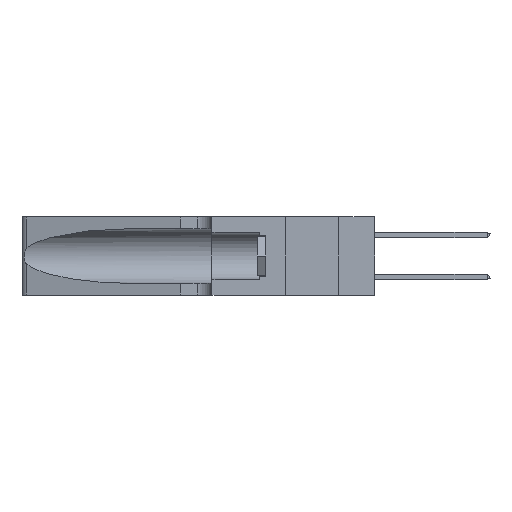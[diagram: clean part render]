
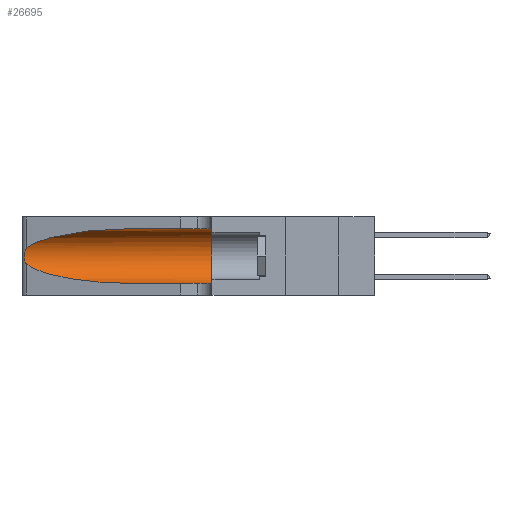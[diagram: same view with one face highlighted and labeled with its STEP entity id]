
A CAD part, left-side view. The second image highlights one B-rep face of the part: STEP entity #26695.
In plain terms, the highlighted cylindrical face has radius 3.308 mm (diameter 6.617 mm), a partial arc.
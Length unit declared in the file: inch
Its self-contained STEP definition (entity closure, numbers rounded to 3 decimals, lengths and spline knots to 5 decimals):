
#45 = VECTOR ( 'NONE', #2268, 39.37008 ) ;
#107 = VERTEX_POINT ( 'NONE', #2009 ) ;
#202 = DIRECTION ( 'NONE',  ( 0., -1., 0. ) ) ;
#942 = CARTESIAN_POINT ( 'NONE',  ( 0.25487, 1.22718, 0.14631 ) ) ;
#1218 = DIRECTION ( 'NONE',  ( 0., 0., 1. ) ) ;
#1444 = CARTESIAN_POINT ( 'NONE',  ( 0.25639, 1.23186, 0.15144 ) ) ;
#2009 = CARTESIAN_POINT ( 'NONE',  ( 0.1305, 0.72297, 0.05475 ) ) ;
#2268 = DIRECTION ( 'NONE',  ( 0., -1., 0. ) ) ;
#2345 = EDGE_CURVE ( 'NONE', #10786, #5442, #5849, .T. ) ;
#3218 = DIRECTION ( 'NONE',  ( 0., 1., 0. ) ) ;
#4179 = EDGE_CURVE ( 'NONE', #23238, #16284, #18968, .T. ) ;
#4226 = ORIENTED_EDGE ( 'NONE', *, *, #7872, .T. ) ;
#5297 = CARTESIAN_POINT ( 'NONE',  ( 0.25787, 1.23484, 0.2124 ) ) ;
#5377 =( BOUNDED_CURVE ( )  B_SPLINE_CURVE ( 3, ( #12181, #7871, #12654, #19190 ),
 .UNSPECIFIED., .F., .T. ) 
 B_SPLINE_CURVE_WITH_KNOTS ( ( 4, 4 ),
 ( 3.44316, 4.71239 ),
 .UNSPECIFIED. ) 
 CURVE ( )  GEOMETRIC_REPRESENTATION_ITEM ( )  RATIONAL_B_SPLINE_CURVE ( ( 1., 0.87, 0.87, 1. ) ) 
 REPRESENTATION_ITEM ( '' )  );
#5442 = VERTEX_POINT ( 'NONE', #18448 ) ;
#5849 = LINE ( 'NONE', #19438, #45 ) ;
#6917 = CARTESIAN_POINT ( 'NONE',  ( 0.25639, 1.23184, 0.21858 ) ) ;
#7208 = CIRCLE ( 'NONE', #15430, 0.13025 ) ;
#7463 = CYLINDRICAL_SURFACE ( 'NONE', #18417, 0.13025 ) ;
#7635 = CARTESIAN_POINT ( 'NONE',  ( 0.26075, 1.23896, 0.19203 ) ) ;
#7871 = CARTESIAN_POINT ( 'NONE',  ( 0.2373, 1.15595, 0.08982 ) ) ;
#7872 = EDGE_CURVE ( 'NONE', #16284, #107, #5377, .T. ) ;
#8431 = DIRECTION ( 'NONE',  ( 0., -1., 0. ) ) ;
#8693 = ORIENTED_EDGE ( 'NONE', *, *, #19929, .T. ) ;
#8828 = CARTESIAN_POINT ( 'NONE',  ( 0.2373, 1.15595, 0.28018 ) ) ;
#10670 = CARTESIAN_POINT ( 'NONE',  ( 0.26018, 1.23835, 0.19895 ) ) ;
#10732 = DIRECTION ( 'NONE',  ( 0., 0., -1. ) ) ;
#10773 = ORIENTED_EDGE ( 'NONE', *, *, #14104, .F. ) ;
#10786 = VERTEX_POINT ( 'NONE', #21447 ) ;
#11016 = EDGE_CURVE ( 'NONE', #10786, #23238, #21423, .T. ) ;
#11410 = VERTEX_POINT ( 'NONE', #18391 ) ;
#12181 = CARTESIAN_POINT ( 'NONE',  ( 0.25487, 1.22718, 0.14631 ) ) ;
#12244 = CARTESIAN_POINT ( 'NONE',  ( 0.25856, 1.23593, 0.16098 ) ) ;
#12654 = CARTESIAN_POINT ( 'NONE',  ( 0.18966, 0.96281, 0.05475 ) ) ;
#12763 = LINE ( 'NONE', #12838, #19871 ) ;
#12838 = CARTESIAN_POINT ( 'NONE',  ( 0.1305, 1.61858, 0.05475 ) ) ;
#13787 = CARTESIAN_POINT ( 'NONE',  ( 0.25854, 1.2359, 0.20912 ) ) ;
#14104 = EDGE_CURVE ( 'NONE', #5442, #11410, #7208, .T. ) ;
#15430 = AXIS2_PLACEMENT_3D ( 'NONE', #20830, #3218, #1218 ) ;
#15683 = CARTESIAN_POINT ( 'NONE',  ( 0.25789, 1.23486, 0.15765 ) ) ;
#16204 = EDGE_LOOP ( 'NONE', ( #25322, #21745, #4226, #8693, #10773, #23568 ) ) ;
#16284 = VERTEX_POINT ( 'NONE', #23345 ) ;
#17478 = CARTESIAN_POINT ( 'NONE',  ( 0.25487, 1.22718, 0.22369 ) ) ;
#18391 = CARTESIAN_POINT ( 'NONE',  ( 0.1305, 0.35, 0.05475 ) ) ;
#18417 = AXIS2_PLACEMENT_3D ( 'NONE', #23978, #202, #10732 ) ;
#18448 = CARTESIAN_POINT ( 'NONE',  ( 0.1305, 0.35, 0.31525 ) ) ;
#18968 = B_SPLINE_CURVE_WITH_KNOTS ( 'NONE', 3,
 ( #19672, #21848, #6917, #5297, #13787, #10670, #7635, #26996, #22846, #12244, #15683, #1444, #24683, #942 ),
 .UNSPECIFIED., .F., .F.,
 ( 4, 2, 2, 2, 2, 2, 4 ),
 ( 0., 0.00027, 0.00053, 0.00107, 0.0016, 0.00187, 0.00214 ),
 .UNSPECIFIED. ) ;
#19190 = CARTESIAN_POINT ( 'NONE',  ( 0.1305, 0.72297, 0.05475 ) ) ;
#19438 = CARTESIAN_POINT ( 'NONE',  ( 0.1305, 1.61858, 0.31525 ) ) ;
#19672 = CARTESIAN_POINT ( 'NONE',  ( 0.25487, 1.22718, 0.22369 ) ) ;
#19871 = VECTOR ( 'NONE', #8431, 39.37008 ) ;
#19929 = EDGE_CURVE ( 'NONE', #107, #11410, #12763, .T. ) ;
#20724 = FACE_OUTER_BOUND ( 'NONE', #16204, .T. ) ;
#20830 = CARTESIAN_POINT ( 'NONE',  ( 0.1305, 0.35, 0.185 ) ) ;
#21423 =( BOUNDED_CURVE ( )  B_SPLINE_CURVE ( 3, ( #23719, #24726, #8828, #17478 ),
 .UNSPECIFIED., .F., .T. ) 
 B_SPLINE_CURVE_WITH_KNOTS ( ( 4, 4 ),
 ( 1.5708, 2.84003 ),
 .UNSPECIFIED. ) 
 CURVE ( )  GEOMETRIC_REPRESENTATION_ITEM ( )  RATIONAL_B_SPLINE_CURVE ( ( 1., 0.87, 0.87, 1. ) ) 
 REPRESENTATION_ITEM ( '' )  );
#21447 = CARTESIAN_POINT ( 'NONE',  ( 0.1305, 0.72297, 0.31525 ) ) ;
#21745 = ORIENTED_EDGE ( 'NONE', *, *, #4179, .T. ) ;
#21848 = CARTESIAN_POINT ( 'NONE',  ( 0.25555, 1.22994, 0.2215 ) ) ;
#22846 = CARTESIAN_POINT ( 'NONE',  ( 0.26017, 1.23833, 0.17102 ) ) ;
#23238 = VERTEX_POINT ( 'NONE', #24776 ) ;
#23345 = CARTESIAN_POINT ( 'NONE',  ( 0.25487, 1.22718, 0.14631 ) ) ;
#23568 = ORIENTED_EDGE ( 'NONE', *, *, #2345, .F. ) ;
#23719 = CARTESIAN_POINT ( 'NONE',  ( 0.1305, 0.72297, 0.31525 ) ) ;
#23978 = CARTESIAN_POINT ( 'NONE',  ( 0.1305, 1.61858, 0.185 ) ) ;
#24683 = CARTESIAN_POINT ( 'NONE',  ( 0.25555, 1.22993, 0.14849 ) ) ;
#24726 = CARTESIAN_POINT ( 'NONE',  ( 0.18966, 0.96281, 0.31525 ) ) ;
#24776 = CARTESIAN_POINT ( 'NONE',  ( 0.25487, 1.22718, 0.22369 ) ) ;
#25322 = ORIENTED_EDGE ( 'NONE', *, *, #11016, .T. ) ;
#26695 = ADVANCED_FACE ( 'NONE', ( #20724 ), #7463, .F. ) ;
#26996 = CARTESIAN_POINT ( 'NONE',  ( 0.26075, 1.23896, 0.178 ) ) ;
